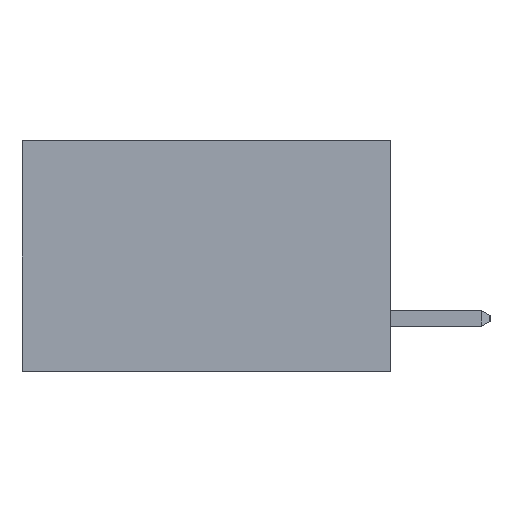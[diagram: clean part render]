
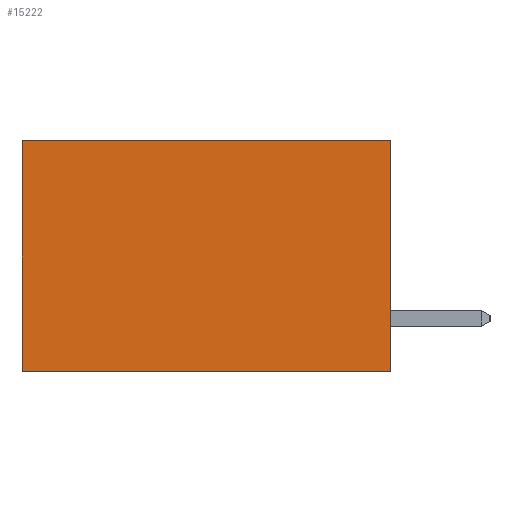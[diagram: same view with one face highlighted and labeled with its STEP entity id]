
A CAD part, left-side view. The second image highlights one B-rep face of the part: STEP entity #15222.
In plain terms, the highlighted planar face has unit normal (-1, 0, 0).
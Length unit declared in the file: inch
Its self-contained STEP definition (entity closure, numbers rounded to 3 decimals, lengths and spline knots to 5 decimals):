
#392 = ORIENTED_EDGE ( 'NONE', *, *, #10828, .F. ) ;
#918 = VECTOR ( 'NONE', #5356, 39.37008 ) ;
#1732 = LINE ( 'NONE', #8559, #9688 ) ;
#2970 = VECTOR ( 'NONE', #12004, 39.37008 ) ;
#3146 = DIRECTION ( 'NONE',  ( 0., 0., -1. ) ) ;
#3492 = ORIENTED_EDGE ( 'NONE', *, *, #4968, .T. ) ;
#3750 = CARTESIAN_POINT ( 'NONE',  ( 0.277, 0.59, -0.37 ) ) ;
#4968 = EDGE_CURVE ( 'NONE', #7771, #11852, #1732, .T. ) ;
#5356 = DIRECTION ( 'NONE',  ( 0., 0., -1. ) ) ;
#5783 = EDGE_CURVE ( 'NONE', #11198, #16954, #15618, .T. ) ;
#7771 = VERTEX_POINT ( 'NONE', #10819 ) ;
#8310 = DIRECTION ( 'NONE',  ( 0., 1., 0. ) ) ;
#8559 = CARTESIAN_POINT ( 'NONE',  ( 0.277, 0., 0. ) ) ;
#9688 = VECTOR ( 'NONE', #8310, 39.37008 ) ;
#9792 = CARTESIAN_POINT ( 'NONE',  ( 0.277, 0., -0.37 ) ) ;
#10020 = VECTOR ( 'NONE', #16792, 39.37008 ) ;
#10449 = EDGE_LOOP ( 'NONE', ( #18754, #13937, #392, #3492 ) ) ;
#10507 = LINE ( 'NONE', #19898, #10020 ) ;
#10819 = CARTESIAN_POINT ( 'NONE',  ( 0.277, 0., 0. ) ) ;
#10828 = EDGE_CURVE ( 'NONE', #7771, #11198, #10507, .T. ) ;
#11055 = CARTESIAN_POINT ( 'NONE',  ( 0.277, 0., -0.37 ) ) ;
#11198 = VERTEX_POINT ( 'NONE', #9792 ) ;
#11852 = VERTEX_POINT ( 'NONE', #20453 ) ;
#12004 = DIRECTION ( 'NONE',  ( 0., 1., 0. ) ) ;
#12073 = CARTESIAN_POINT ( 'NONE',  ( 0.277, 0., -0.37 ) ) ;
#12638 = DIRECTION ( 'NONE',  ( 1., 0., 0. ) ) ;
#13937 = ORIENTED_EDGE ( 'NONE', *, *, #5783, .F. ) ;
#14026 = EDGE_CURVE ( 'NONE', #11852, #16954, #17297, .T. ) ;
#14721 = AXIS2_PLACEMENT_3D ( 'NONE', #11055, #12638, #3146 ) ;
#15222 = ADVANCED_FACE ( 'NONE', ( #19658 ), #20462, .F. ) ;
#15618 = LINE ( 'NONE', #12073, #2970 ) ;
#16792 = DIRECTION ( 'NONE',  ( 0., 0., -1. ) ) ;
#16954 = VERTEX_POINT ( 'NONE', #20057 ) ;
#17297 = LINE ( 'NONE', #3750, #918 ) ;
#18754 = ORIENTED_EDGE ( 'NONE', *, *, #14026, .T. ) ;
#19658 = FACE_OUTER_BOUND ( 'NONE', #10449, .T. ) ;
#19898 = CARTESIAN_POINT ( 'NONE',  ( 0.277, 0., -0.37 ) ) ;
#20057 = CARTESIAN_POINT ( 'NONE',  ( 0.277, 0.59, -0.37 ) ) ;
#20453 = CARTESIAN_POINT ( 'NONE',  ( 0.277, 0.59, 0. ) ) ;
#20462 = PLANE ( 'NONE',  #14721 ) ;
